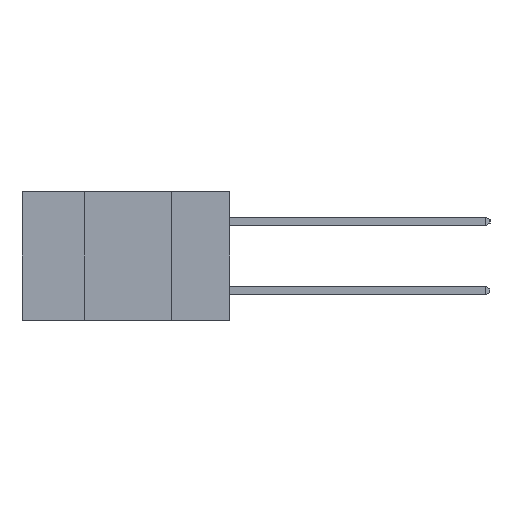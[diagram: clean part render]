
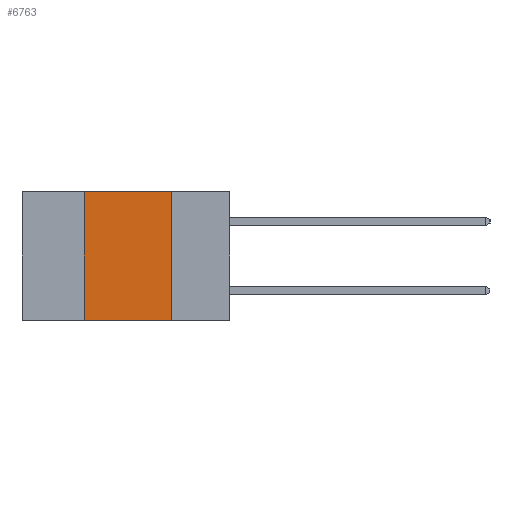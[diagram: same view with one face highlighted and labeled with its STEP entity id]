
A CAD part, left-side view. The second image highlights one B-rep face of the part: STEP entity #6763.
In plain terms, the highlighted planar face has unit normal (-1, 0, 0).
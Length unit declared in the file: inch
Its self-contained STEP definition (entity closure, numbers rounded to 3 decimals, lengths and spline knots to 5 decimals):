
#154 = VERTEX_POINT ( 'NONE', #18804 ) ;
#2322 = CARTESIAN_POINT ( 'NONE',  ( 0., 0.6, 0. ) ) ;
#2745 = DIRECTION ( 'NONE',  ( 0., 0., 1. ) ) ;
#3607 = VECTOR ( 'NONE', #2745, 39.37008 ) ;
#4374 = DIRECTION ( 'NONE',  ( 0., -1., 0. ) ) ;
#4822 = CARTESIAN_POINT ( 'NONE',  ( 0., 0.17, -0.37 ) ) ;
#6051 = ORIENTED_EDGE ( 'NONE', *, *, #10937, .F. ) ;
#6589 = LINE ( 'NONE', #2322, #16899 ) ;
#6763 = ADVANCED_FACE ( 'NONE', ( #17706 ), #10131, .F. ) ;
#8117 = AXIS2_PLACEMENT_3D ( 'NONE', #24483, #26555, #14286 ) ;
#8887 = CARTESIAN_POINT ( 'NONE',  ( 0., 0.6, -0.37 ) ) ;
#9012 = EDGE_LOOP ( 'NONE', ( #13159, #22786, #6051, #26636 ) ) ;
#9358 = VERTEX_POINT ( 'NONE', #20128 ) ;
#9734 = EDGE_CURVE ( 'NONE', #154, #25340, #21756, .T. ) ;
#9977 = DIRECTION ( 'NONE',  ( 0., 0., -1. ) ) ;
#10131 = PLANE ( 'NONE',  #8117 ) ;
#10937 = EDGE_CURVE ( 'NONE', #154, #9358, #25519, .T. ) ;
#11263 = EDGE_CURVE ( 'NONE', #21088, #25340, #13011, .T. ) ;
#13011 = LINE ( 'NONE', #20224, #23269 ) ;
#13159 = ORIENTED_EDGE ( 'NONE', *, *, #11263, .F. ) ;
#14286 = DIRECTION ( 'NONE',  ( 0., 0., -1. ) ) ;
#15085 = DIRECTION ( 'NONE',  ( 0., -1., 0. ) ) ;
#15213 = CARTESIAN_POINT ( 'NONE',  ( 0., 0.42, -0.37 ) ) ;
#16300 = VECTOR ( 'NONE', #15085, 39.37008 ) ;
#16402 = CARTESIAN_POINT ( 'NONE',  ( 0., 0.17, 0. ) ) ;
#16899 = VECTOR ( 'NONE', #4374, 39.37008 ) ;
#17706 = FACE_OUTER_BOUND ( 'NONE', #9012, .T. ) ;
#18804 = CARTESIAN_POINT ( 'NONE',  ( 0., 0.42, -0.37 ) ) ;
#20128 = CARTESIAN_POINT ( 'NONE',  ( 0., 0.42, 0. ) ) ;
#20224 = CARTESIAN_POINT ( 'NONE',  ( 0., 0.17, -0.37 ) ) ;
#21088 = VERTEX_POINT ( 'NONE', #16402 ) ;
#21756 = LINE ( 'NONE', #8887, #16300 ) ;
#22786 = ORIENTED_EDGE ( 'NONE', *, *, #23868, .F. ) ;
#23269 = VECTOR ( 'NONE', #9977, 39.37008 ) ;
#23868 = EDGE_CURVE ( 'NONE', #9358, #21088, #6589, .T. ) ;
#24483 = CARTESIAN_POINT ( 'NONE',  ( 0., 0.6, 0. ) ) ;
#25340 = VERTEX_POINT ( 'NONE', #4822 ) ;
#25519 = LINE ( 'NONE', #15213, #3607 ) ;
#26555 = DIRECTION ( 'NONE',  ( 1., 0., 0. ) ) ;
#26636 = ORIENTED_EDGE ( 'NONE', *, *, #9734, .T. ) ;
